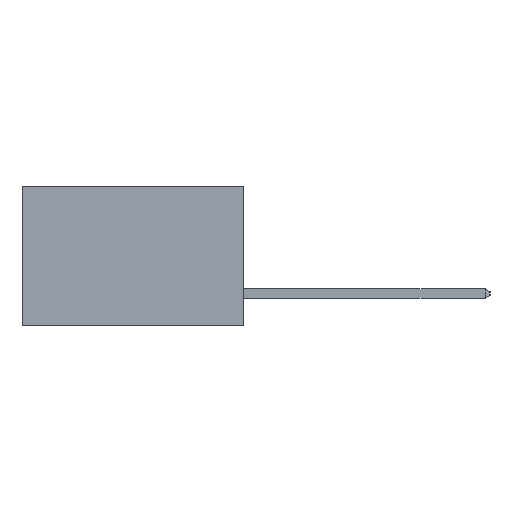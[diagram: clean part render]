
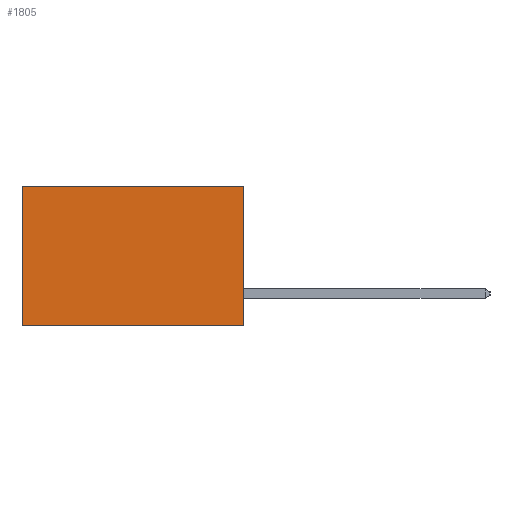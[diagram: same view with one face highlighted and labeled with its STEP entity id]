
A CAD part, left-side view. The second image highlights one B-rep face of the part: STEP entity #1805.
In plain terms, the highlighted planar face has unit normal (-1, 0, 0).
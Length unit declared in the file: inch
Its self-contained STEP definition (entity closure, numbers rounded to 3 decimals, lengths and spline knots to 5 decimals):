
#963 = CARTESIAN_POINT ( 'NONE',  ( 0.277, 0., -0.37 ) ) ;
#1110 = EDGE_LOOP ( 'NONE', ( #9461, #3812, #1603, #14698 ) ) ;
#1138 = LINE ( 'NONE', #4509, #9170 ) ;
#1286 = CARTESIAN_POINT ( 'NONE',  ( 0.277, 0., -0.37 ) ) ;
#1603 = ORIENTED_EDGE ( 'NONE', *, *, #14572, .F. ) ;
#1805 = ADVANCED_FACE ( 'NONE', ( #8421 ), #12154, .F. ) ;
#2274 = CARTESIAN_POINT ( 'NONE',  ( 0.277, 0., 0. ) ) ;
#3260 = CARTESIAN_POINT ( 'NONE',  ( 0.277, 0.59, -0.37 ) ) ;
#3622 = CARTESIAN_POINT ( 'NONE',  ( 0.277, 0., 0. ) ) ;
#3812 = ORIENTED_EDGE ( 'NONE', *, *, #12488, .F. ) ;
#4506 = VECTOR ( 'NONE', #13191, 39.37008 ) ;
#4509 = CARTESIAN_POINT ( 'NONE',  ( 0.277, 0., -0.37 ) ) ;
#5204 = CARTESIAN_POINT ( 'NONE',  ( 0.277, 0.59, -0.37 ) ) ;
#5451 = VERTEX_POINT ( 'NONE', #12252 ) ;
#6510 = VERTEX_POINT ( 'NONE', #3260 ) ;
#6904 = VECTOR ( 'NONE', #11167, 39.37008 ) ;
#7141 = VERTEX_POINT ( 'NONE', #3622 ) ;
#8421 = FACE_OUTER_BOUND ( 'NONE', #1110, .T. ) ;
#9170 = VECTOR ( 'NONE', #17672, 39.37008 ) ;
#9312 = LINE ( 'NONE', #2274, #16525 ) ;
#9461 = ORIENTED_EDGE ( 'NONE', *, *, #9685, .T. ) ;
#9685 = EDGE_CURVE ( 'NONE', #5451, #6510, #14665, .T. ) ;
#10902 = DIRECTION ( 'NONE',  ( 1., 0., 0. ) ) ;
#11167 = DIRECTION ( 'NONE',  ( 0., 0., -1. ) ) ;
#12154 = PLANE ( 'NONE',  #13470 ) ;
#12252 = CARTESIAN_POINT ( 'NONE',  ( 0.277, 0.59, 0. ) ) ;
#12488 = EDGE_CURVE ( 'NONE', #15095, #6510, #16206, .T. ) ;
#13094 = CARTESIAN_POINT ( 'NONE',  ( 0.277, 0., -0.37 ) ) ;
#13191 = DIRECTION ( 'NONE',  ( 0., 1., 0. ) ) ;
#13470 = AXIS2_PLACEMENT_3D ( 'NONE', #963, #10902, #15610 ) ;
#14122 = DIRECTION ( 'NONE',  ( 0., 1., 0. ) ) ;
#14572 = EDGE_CURVE ( 'NONE', #7141, #15095, #1138, .T. ) ;
#14665 = LINE ( 'NONE', #5204, #6904 ) ;
#14698 = ORIENTED_EDGE ( 'NONE', *, *, #18325, .T. ) ;
#15095 = VERTEX_POINT ( 'NONE', #13094 ) ;
#15610 = DIRECTION ( 'NONE',  ( 0., 0., -1. ) ) ;
#16206 = LINE ( 'NONE', #1286, #4506 ) ;
#16525 = VECTOR ( 'NONE', #14122, 39.37008 ) ;
#17672 = DIRECTION ( 'NONE',  ( 0., 0., -1. ) ) ;
#18325 = EDGE_CURVE ( 'NONE', #7141, #5451, #9312, .T. ) ;
